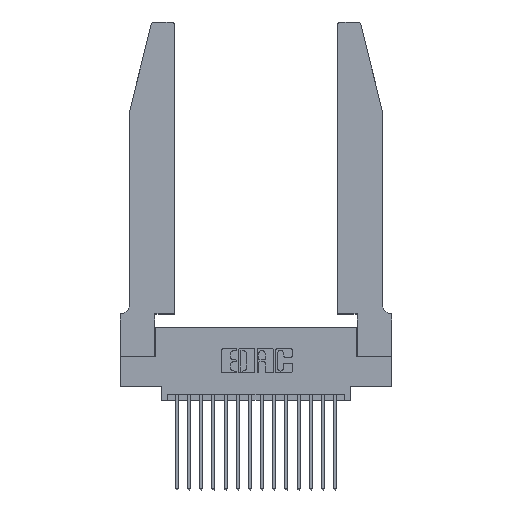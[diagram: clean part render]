
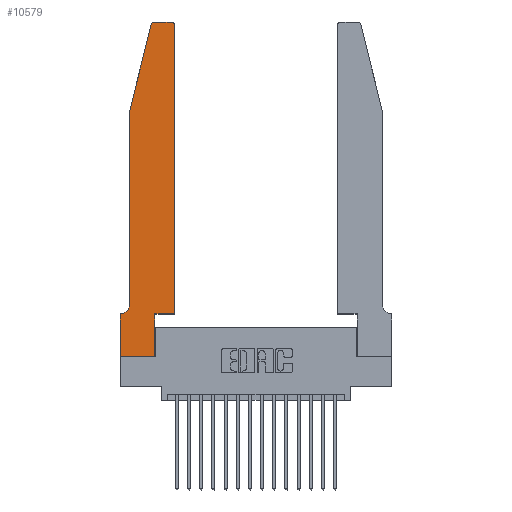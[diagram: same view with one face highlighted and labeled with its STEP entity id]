
A CAD part, top view. The second image highlights one B-rep face of the part: STEP entity #10579.
In plain terms, the highlighted planar face has unit normal (0, 0, 1).
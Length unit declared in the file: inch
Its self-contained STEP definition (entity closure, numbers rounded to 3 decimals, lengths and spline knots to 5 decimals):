
#37 = VERTEX_POINT ( 'NONE', #15666 ) ;
#124 = VERTEX_POINT ( 'NONE', #15060 ) ;
#150 = CARTESIAN_POINT ( 'NONE',  ( 0.0755, 0.35, 0.37 ) ) ;
#163 = ORIENTED_EDGE ( 'NONE', *, *, #5346, .T. ) ;
#655 = CARTESIAN_POINT ( 'NONE',  ( 0.2865, 0.35, 0.37 ) ) ;
#1253 = CIRCLE ( 'NONE', #19151, 0.03 ) ;
#1257 = DIRECTION ( 'NONE',  ( 1., 0., 0. ) ) ;
#1522 = VERTEX_POINT ( 'NONE', #17854 ) ;
#1660 = LINE ( 'NONE', #1718, #9879 ) ;
#1718 = CARTESIAN_POINT ( 'NONE',  ( 0.2605, 2.75, 0.37 ) ) ;
#2220 = DIRECTION ( 'NONE',  ( 1., 0., 0. ) ) ;
#2390 = AXIS2_PLACEMENT_3D ( 'NONE', #17883, #10516, #1257 ) ;
#2785 = PLANE ( 'NONE',  #2390 ) ;
#2901 = VECTOR ( 'NONE', #14453, 39.37008 ) ;
#2988 = EDGE_CURVE ( 'NONE', #124, #4469, #7115, .T. ) ;
#3015 = AXIS2_PLACEMENT_3D ( 'NONE', #13828, #4765, #15295 ) ;
#3052 = LINE ( 'NONE', #12940, #13778 ) ;
#3378 = ORIENTED_EDGE ( 'NONE', *, *, #8769, .T. ) ;
#3390 = CIRCLE ( 'NONE', #7330, 0.03 ) ;
#3626 = VECTOR ( 'NONE', #15431, 39.37008 ) ;
#3995 = ORIENTED_EDGE ( 'NONE', *, *, #19616, .T. ) ;
#4191 = DIRECTION ( 'NONE',  ( 0., 0., 1. ) ) ;
#4469 = VERTEX_POINT ( 'NONE', #19215 ) ;
#4530 = ORIENTED_EDGE ( 'NONE', *, *, #12469, .T. ) ;
#4765 = DIRECTION ( 'NONE',  ( 0., 0., -1. ) ) ;
#4775 = EDGE_CURVE ( 'NONE', #12299, #9400, #17464, .T. ) ;
#4783 = VECTOR ( 'NONE', #10719, 39.37008 ) ;
#4916 = CARTESIAN_POINT ( 'NONE',  ( 0., 0., 0.37 ) ) ;
#5067 = VERTEX_POINT ( 'NONE', #14540 ) ;
#5244 = VERTEX_POINT ( 'NONE', #13592 ) ;
#5346 = EDGE_CURVE ( 'NONE', #19266, #12299, #9065, .T. ) ;
#6111 = FACE_OUTER_BOUND ( 'NONE', #8932, .T. ) ;
#6435 = DIRECTION ( 'NONE',  ( -1., 0., 0. ) ) ;
#6551 = CARTESIAN_POINT ( 'NONE',  ( 0.4505, 0.35, 0.37 ) ) ;
#7019 = CARTESIAN_POINT ( 'NONE',  ( 0.0755, 2., 0.37 ) ) ;
#7115 = LINE ( 'NONE', #655, #18538 ) ;
#7313 = VECTOR ( 'NONE', #7675, 39.37008 ) ;
#7330 = AXIS2_PLACEMENT_3D ( 'NONE', #13303, #4191, #14762 ) ;
#7675 = DIRECTION ( 'NONE',  ( -0.239, -0.971, 0. ) ) ;
#7728 = CARTESIAN_POINT ( 'NONE',  ( 0., 0., 0.37 ) ) ;
#7927 = ORIENTED_EDGE ( 'NONE', *, *, #10080, .T. ) ;
#7939 = ORIENTED_EDGE ( 'NONE', *, *, #14541, .T. ) ;
#8087 = CARTESIAN_POINT ( 'NONE',  ( 0.4205, 2.72, 0.37 ) ) ;
#8137 = CARTESIAN_POINT ( 'NONE',  ( 0.4205, 2.75, 0.37 ) ) ;
#8243 = ORIENTED_EDGE ( 'NONE', *, *, #11315, .T. ) ;
#8719 = ORIENTED_EDGE ( 'NONE', *, *, #4775, .T. ) ;
#8769 = EDGE_CURVE ( 'NONE', #5244, #5067, #14369, .T. ) ;
#8932 = EDGE_LOOP ( 'NONE', ( #8243, #16147, #3378, #16945, #163, #8719, #7939, #4530, #12137, #15710, #7927, #3995 ) ) ;
#9065 = CIRCLE ( 'NONE', #3015, 0.07 ) ;
#9124 = CARTESIAN_POINT ( 'NONE',  ( 0.4505, 0.35, 0.37 ) ) ;
#9400 = VERTEX_POINT ( 'NONE', #12089 ) ;
#9566 = VECTOR ( 'NONE', #6435, 39.37008 ) ;
#9613 = DIRECTION ( 'NONE',  ( 1., 0., 0. ) ) ;
#9879 = VECTOR ( 'NONE', #16949, 39.37008 ) ;
#9901 = CARTESIAN_POINT ( 'NONE',  ( 0.0755, 0.42, 0.37 ) ) ;
#9923 = EDGE_CURVE ( 'NONE', #37, #5244, #3390, .T. ) ;
#9952 = DIRECTION ( 'NONE',  ( 0., 1., 0. ) ) ;
#10080 = EDGE_CURVE ( 'NONE', #17644, #1522, #12712, .T. ) ;
#10516 = DIRECTION ( 'NONE',  ( 0., 0., 1. ) ) ;
#10579 = ADVANCED_FACE ( 'NONE', ( #6111 ), #2785, .T. ) ;
#10719 = DIRECTION ( 'NONE',  ( 0., -1., 0. ) ) ;
#11315 = EDGE_CURVE ( 'NONE', #17700, #37, #1660, .T. ) ;
#11479 = EDGE_CURVE ( 'NONE', #5067, #19266, #15459, .T. ) ;
#12089 = CARTESIAN_POINT ( 'NONE',  ( 0., 0.35, 0.37 ) ) ;
#12137 = ORIENTED_EDGE ( 'NONE', *, *, #2988, .T. ) ;
#12299 = VERTEX_POINT ( 'NONE', #13607 ) ;
#12469 = EDGE_CURVE ( 'NONE', #16868, #124, #18663, .T. ) ;
#12712 = LINE ( 'NONE', #9124, #17066 ) ;
#12940 = CARTESIAN_POINT ( 'NONE',  ( 0.4505, 0.35, 0.37 ) ) ;
#13303 = CARTESIAN_POINT ( 'NONE',  ( 0.284, 2.72, 0.37 ) ) ;
#13328 = LINE ( 'NONE', #7728, #4783 ) ;
#13592 = CARTESIAN_POINT ( 'NONE',  ( 0.25487, 2.72718, 0.37 ) ) ;
#13607 = CARTESIAN_POINT ( 'NONE',  ( 0.0055, 0.35, 0.37 ) ) ;
#13778 = VECTOR ( 'NONE', #2220, 39.37008 ) ;
#13828 = CARTESIAN_POINT ( 'NONE',  ( 0.0055, 0.42, 0.37 ) ) ;
#14369 = LINE ( 'NONE', #16602, #7313 ) ;
#14453 = DIRECTION ( 'NONE',  ( 0., -1., 0. ) ) ;
#14540 = CARTESIAN_POINT ( 'NONE',  ( 0.0755, 2., 0.37 ) ) ;
#14541 = EDGE_CURVE ( 'NONE', #9400, #16868, #13328, .T. ) ;
#14762 = DIRECTION ( 'NONE',  ( 1., 0., 0. ) ) ;
#15060 = CARTESIAN_POINT ( 'NONE',  ( 0.2865, 0., 0.37 ) ) ;
#15295 = DIRECTION ( 'NONE',  ( -1., 0., 0. ) ) ;
#15431 = DIRECTION ( 'NONE',  ( 1., 0., 0. ) ) ;
#15459 = LINE ( 'NONE', #7019, #2901 ) ;
#15666 = CARTESIAN_POINT ( 'NONE',  ( 0.284, 2.75, 0.37 ) ) ;
#15710 = ORIENTED_EDGE ( 'NONE', *, *, #18422, .T. ) ;
#16147 = ORIENTED_EDGE ( 'NONE', *, *, #9923, .T. ) ;
#16602 = CARTESIAN_POINT ( 'NONE',  ( 0.0755, 2., 0.37 ) ) ;
#16701 = CARTESIAN_POINT ( 'NONE',  ( 0., 0., 0.37 ) ) ;
#16868 = VERTEX_POINT ( 'NONE', #16701 ) ;
#16945 = ORIENTED_EDGE ( 'NONE', *, *, #11479, .T. ) ;
#16949 = DIRECTION ( 'NONE',  ( -1., 0., 0. ) ) ;
#17066 = VECTOR ( 'NONE', #19515, 39.37008 ) ;
#17464 = LINE ( 'NONE', #150, #9566 ) ;
#17644 = VERTEX_POINT ( 'NONE', #6551 ) ;
#17700 = VERTEX_POINT ( 'NONE', #8137 ) ;
#17854 = CARTESIAN_POINT ( 'NONE',  ( 0.4505, 2.72, 0.37 ) ) ;
#17883 = CARTESIAN_POINT ( 'NONE',  ( 0., 0.35, 0.37 ) ) ;
#18422 = EDGE_CURVE ( 'NONE', #4469, #17644, #3052, .T. ) ;
#18490 = DIRECTION ( 'NONE',  ( 0., 0., 1. ) ) ;
#18538 = VECTOR ( 'NONE', #9952, 39.37008 ) ;
#18663 = LINE ( 'NONE', #4916, #3626 ) ;
#19151 = AXIS2_PLACEMENT_3D ( 'NONE', #8087, #18490, #9613 ) ;
#19215 = CARTESIAN_POINT ( 'NONE',  ( 0.2865, 0.35, 0.37 ) ) ;
#19266 = VERTEX_POINT ( 'NONE', #9901 ) ;
#19515 = DIRECTION ( 'NONE',  ( 0., 1., 0. ) ) ;
#19616 = EDGE_CURVE ( 'NONE', #1522, #17700, #1253, .T. ) ;
